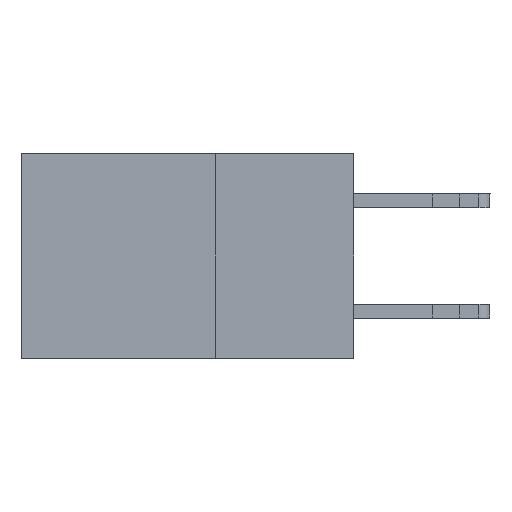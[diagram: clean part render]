
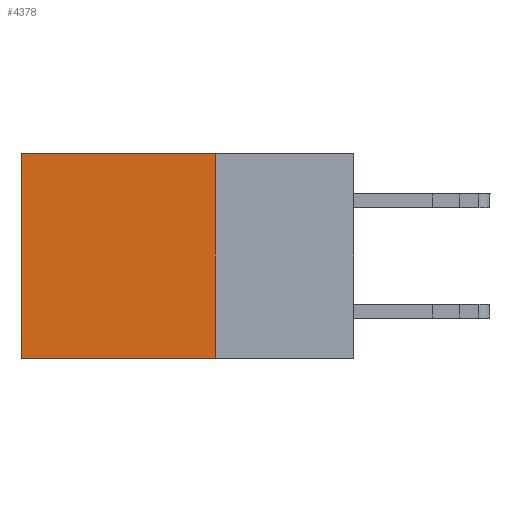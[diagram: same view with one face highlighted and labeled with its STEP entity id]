
A CAD part, left-side view. The second image highlights one B-rep face of the part: STEP entity #4378.
In plain terms, the highlighted planar face has unit normal (-1, 0, 0).
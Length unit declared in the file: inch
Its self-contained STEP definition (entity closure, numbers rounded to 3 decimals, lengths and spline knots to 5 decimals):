
#217 = LINE ( 'NONE', #24092, #20028 ) ;
#335 = CARTESIAN_POINT ( 'NONE',  ( 0.2875, 0.6, -0.37 ) ) ;
#455 = PLANE ( 'NONE',  #2946 ) ;
#911 = EDGE_LOOP ( 'NONE', ( #20994, #16483, #10002, #24666 ) ) ;
#1438 = VERTEX_POINT ( 'NONE', #15631 ) ;
#1478 = DIRECTION ( 'NONE',  ( 0., 1., 0. ) ) ;
#2152 = CARTESIAN_POINT ( 'NONE',  ( 0.2875, 0.25, 0. ) ) ;
#2444 = CARTESIAN_POINT ( 'NONE',  ( 0.2875, 0.25, 0. ) ) ;
#2482 = DIRECTION ( 'NONE',  ( 0., 0., -1. ) ) ;
#2946 = AXIS2_PLACEMENT_3D ( 'NONE', #10342, #14327, #2482 ) ;
#4179 = VERTEX_POINT ( 'NONE', #7776 ) ;
#4378 = ADVANCED_FACE ( 'NONE', ( #8737 ), #455, .F. ) ;
#4608 = LINE ( 'NONE', #11336, #14498 ) ;
#4943 = CARTESIAN_POINT ( 'NONE',  ( 0.2875, 0.25, -0.37 ) ) ;
#7776 = CARTESIAN_POINT ( 'NONE',  ( 0.2875, 0.6, 0. ) ) ;
#8737 = FACE_OUTER_BOUND ( 'NONE', #911, .T. ) ;
#10002 = ORIENTED_EDGE ( 'NONE', *, *, #20665, .F. ) ;
#10016 = LINE ( 'NONE', #2444, #25160 ) ;
#10342 = CARTESIAN_POINT ( 'NONE',  ( 0.2875, 0.25, 0. ) ) ;
#11336 = CARTESIAN_POINT ( 'NONE',  ( 0.2875, 0.25, -0.37 ) ) ;
#11455 = VERTEX_POINT ( 'NONE', #4943 ) ;
#13595 = VERTEX_POINT ( 'NONE', #335 ) ;
#14327 = DIRECTION ( 'NONE',  ( 1., 0., 0. ) ) ;
#14498 = VECTOR ( 'NONE', #1478, 39.37008 ) ;
#15631 = CARTESIAN_POINT ( 'NONE',  ( 0.2875, 0.25, 0. ) ) ;
#16483 = ORIENTED_EDGE ( 'NONE', *, *, #17895, .F. ) ;
#17455 = VECTOR ( 'NONE', #21801, 39.37008 ) ;
#17895 = EDGE_CURVE ( 'NONE', #11455, #13595, #4608, .T. ) ;
#18078 = EDGE_CURVE ( 'NONE', #4179, #13595, #217, .T. ) ;
#18093 = LINE ( 'NONE', #2152, #17455 ) ;
#18247 = DIRECTION ( 'NONE',  ( 0., 1., 0. ) ) ;
#20028 = VECTOR ( 'NONE', #20211, 39.37008 ) ;
#20211 = DIRECTION ( 'NONE',  ( 0., 0., -1. ) ) ;
#20665 = EDGE_CURVE ( 'NONE', #1438, #11455, #18093, .T. ) ;
#20994 = ORIENTED_EDGE ( 'NONE', *, *, #18078, .T. ) ;
#21801 = DIRECTION ( 'NONE',  ( 0., 0., -1. ) ) ;
#24092 = CARTESIAN_POINT ( 'NONE',  ( 0.2875, 0.6, 0. ) ) ;
#24666 = ORIENTED_EDGE ( 'NONE', *, *, #25611, .T. ) ;
#25160 = VECTOR ( 'NONE', #18247, 39.37008 ) ;
#25611 = EDGE_CURVE ( 'NONE', #1438, #4179, #10016, .T. ) ;
